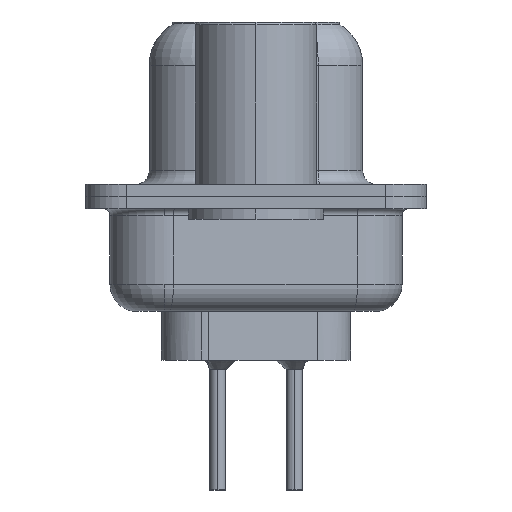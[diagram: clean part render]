
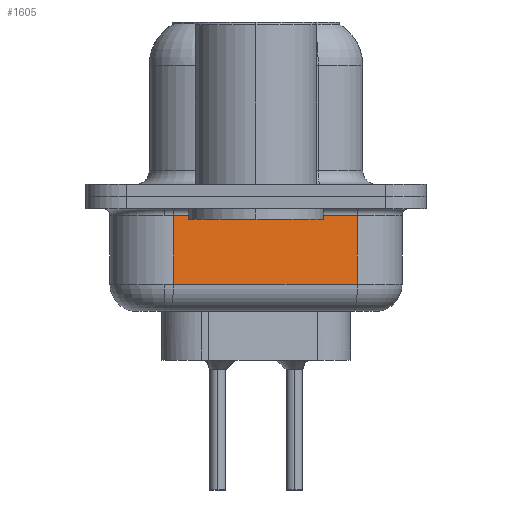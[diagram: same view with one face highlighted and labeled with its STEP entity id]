
A CAD part, left-side view. The second image highlights one B-rep face of the part: STEP entity #1605.
In plain terms, the highlighted planar face has unit normal (-0.985, -0.174, 0).
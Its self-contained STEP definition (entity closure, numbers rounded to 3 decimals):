
#138 = CARTESIAN_POINT ( 'NONE',  ( 2.89, 3.053, -0.7 ) ) ;
#531 = CARTESIAN_POINT ( 'NONE',  ( 2.89, 3.053, -3.25 ) ) ;
#1165 = VECTOR ( 'NONE', #24655, 1000. ) ;
#1605 = ADVANCED_FACE ( 'NONE', ( #8972 ), #20785, .F. ) ;
#1641 = CARTESIAN_POINT ( 'NONE',  ( 2.89, 3.053, -4.25 ) ) ;
#1864 = LINE ( 'NONE', #13330, #1165 ) ;
#1944 = VERTEX_POINT ( 'NONE', #18613 ) ;
#3203 = VERTEX_POINT ( 'NONE', #13770 ) ;
#3368 = ORIENTED_EDGE ( 'NONE', *, *, #15810, .T. ) ;
#4985 = ORIENTED_EDGE ( 'NONE', *, *, #10469, .T. ) ;
#5471 = EDGE_LOOP ( 'NONE', ( #7262, #4985, #3368, #6679 ) ) ;
#5941 = CARTESIAN_POINT ( 'NONE',  ( 2.89, 3.053, -0.7 ) ) ;
#6679 = ORIENTED_EDGE ( 'NONE', *, *, #22009, .T. ) ;
#7079 = VERTEX_POINT ( 'NONE', #5941 ) ;
#7262 = ORIENTED_EDGE ( 'NONE', *, *, #18217, .F. ) ;
#7978 = LINE ( 'NONE', #531, #11956 ) ;
#8213 = LINE ( 'NONE', #138, #10117 ) ;
#8972 = FACE_OUTER_BOUND ( 'NONE', #5471, .T. ) ;
#9098 = DIRECTION ( 'NONE',  ( -0.174, 0.985, 0. ) ) ;
#9286 = VECTOR ( 'NONE', #20476, 1000. ) ;
#9344 = DIRECTION ( 'NONE',  ( 0.985, 0.174, 0. ) ) ;
#9868 = DIRECTION ( 'NONE',  ( -0.174, 0.985, 0. ) ) ;
#10117 = VECTOR ( 'NONE', #9868, 1000. ) ;
#10469 = EDGE_CURVE ( 'NONE', #1944, #3203, #7978, .T. ) ;
#10661 = CARTESIAN_POINT ( 'NONE',  ( 4.089, -3.747, -4.25 ) ) ;
#11765 = DIRECTION ( 'NONE',  ( 0.174, -0.985, 0. ) ) ;
#11956 = VECTOR ( 'NONE', #11765, 1000. ) ;
#12346 = VERTEX_POINT ( 'NONE', #22504 ) ;
#12800 = LINE ( 'NONE', #10661, #9286 ) ;
#13330 = CARTESIAN_POINT ( 'NONE',  ( 2.89, 3.053, -4.25 ) ) ;
#13770 = CARTESIAN_POINT ( 'NONE',  ( 4.089, -3.747, -3.25 ) ) ;
#14149 = AXIS2_PLACEMENT_3D ( 'NONE', #1641, #9344, #9098 ) ;
#15810 = EDGE_CURVE ( 'NONE', #3203, #12346, #12800, .T. ) ;
#18217 = EDGE_CURVE ( 'NONE', #1944, #7079, #1864, .T. ) ;
#18613 = CARTESIAN_POINT ( 'NONE',  ( 2.89, 3.053, -3.25 ) ) ;
#20476 = DIRECTION ( 'NONE',  ( 0., 0., 1. ) ) ;
#20785 = PLANE ( 'NONE',  #14149 ) ;
#22009 = EDGE_CURVE ( 'NONE', #12346, #7079, #8213, .T. ) ;
#22504 = CARTESIAN_POINT ( 'NONE',  ( 4.089, -3.747, -0.7 ) ) ;
#24655 = DIRECTION ( 'NONE',  ( 0., 0., 1. ) ) ;
